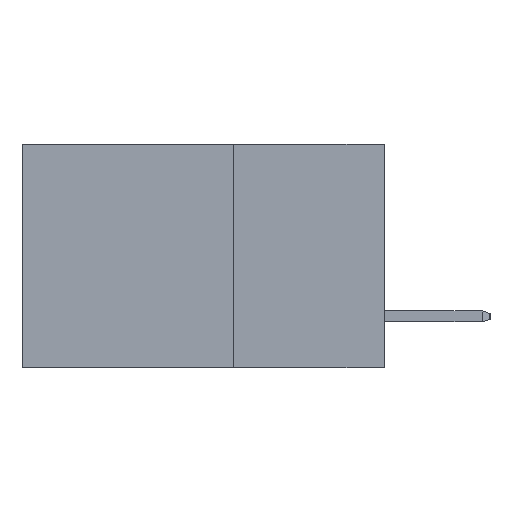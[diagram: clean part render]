
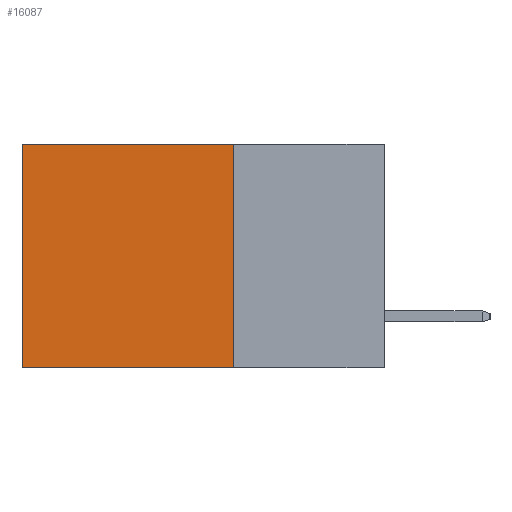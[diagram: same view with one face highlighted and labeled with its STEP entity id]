
A CAD part, left-side view. The second image highlights one B-rep face of the part: STEP entity #16087.
In plain terms, the highlighted planar face has unit normal (-1, 0, 0).
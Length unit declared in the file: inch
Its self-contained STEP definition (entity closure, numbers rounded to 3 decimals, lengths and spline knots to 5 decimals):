
#311 = CARTESIAN_POINT ( 'NONE',  ( 0.298, 0.6, -0.37 ) ) ;
#417 = VERTEX_POINT ( 'NONE', #12931 ) ;
#874 = LINE ( 'NONE', #2561, #19505 ) ;
#1099 = CARTESIAN_POINT ( 'NONE',  ( 0.298, 0.25, 0. ) ) ;
#1668 = ORIENTED_EDGE ( 'NONE', *, *, #6277, .T. ) ;
#1771 = ORIENTED_EDGE ( 'NONE', *, *, #13602, .F. ) ;
#1777 = VECTOR ( 'NONE', #9211, 39.37008 ) ;
#2102 = CARTESIAN_POINT ( 'NONE',  ( 0.298, 0.25, 0. ) ) ;
#2561 = CARTESIAN_POINT ( 'NONE',  ( 0.298, 0.25, 0. ) ) ;
#3713 = PLANE ( 'NONE',  #12067 ) ;
#4642 = DIRECTION ( 'NONE',  ( 0., 1., 0. ) ) ;
#4766 = VERTEX_POINT ( 'NONE', #5437 ) ;
#5437 = CARTESIAN_POINT ( 'NONE',  ( 0.298, 0.6, 0. ) ) ;
#5632 = DIRECTION ( 'NONE',  ( 0., 0., -1. ) ) ;
#6254 = EDGE_LOOP ( 'NONE', ( #12022, #13083, #1771, #1668 ) ) ;
#6277 = EDGE_CURVE ( 'NONE', #417, #4766, #7948, .T. ) ;
#6395 = LINE ( 'NONE', #16327, #15723 ) ;
#6961 = FACE_OUTER_BOUND ( 'NONE', #6254, .T. ) ;
#7040 = LINE ( 'NONE', #17910, #1777 ) ;
#7948 = LINE ( 'NONE', #1099, #16681 ) ;
#9211 = DIRECTION ( 'NONE',  ( 0., 1., 0. ) ) ;
#11416 = EDGE_CURVE ( 'NONE', #16923, #15436, #7040, .T. ) ;
#12022 = ORIENTED_EDGE ( 'NONE', *, *, #16803, .T. ) ;
#12067 = AXIS2_PLACEMENT_3D ( 'NONE', #2102, #16140, #5632 ) ;
#12805 = DIRECTION ( 'NONE',  ( 0., 0., -1. ) ) ;
#12931 = CARTESIAN_POINT ( 'NONE',  ( 0.298, 0.25, 0. ) ) ;
#13083 = ORIENTED_EDGE ( 'NONE', *, *, #11416, .F. ) ;
#13602 = EDGE_CURVE ( 'NONE', #417, #16923, #874, .T. ) ;
#14845 = DIRECTION ( 'NONE',  ( 0., 0., -1. ) ) ;
#15436 = VERTEX_POINT ( 'NONE', #311 ) ;
#15723 = VECTOR ( 'NONE', #12805, 39.37008 ) ;
#16087 = ADVANCED_FACE ( 'NONE', ( #6961 ), #3713, .F. ) ;
#16140 = DIRECTION ( 'NONE',  ( 1., 0., 0. ) ) ;
#16327 = CARTESIAN_POINT ( 'NONE',  ( 0.298, 0.6, 0. ) ) ;
#16681 = VECTOR ( 'NONE', #4642, 39.37008 ) ;
#16803 = EDGE_CURVE ( 'NONE', #4766, #15436, #6395, .T. ) ;
#16923 = VERTEX_POINT ( 'NONE', #21869 ) ;
#17910 = CARTESIAN_POINT ( 'NONE',  ( 0.298, 0.25, -0.37 ) ) ;
#19505 = VECTOR ( 'NONE', #14845, 39.37008 ) ;
#21869 = CARTESIAN_POINT ( 'NONE',  ( 0.298, 0.25, -0.37 ) ) ;
